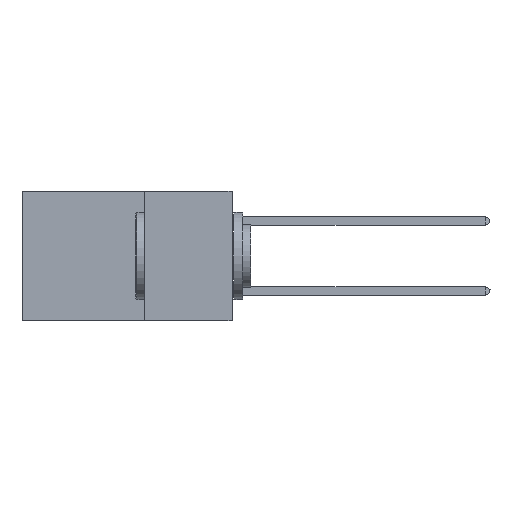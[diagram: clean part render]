
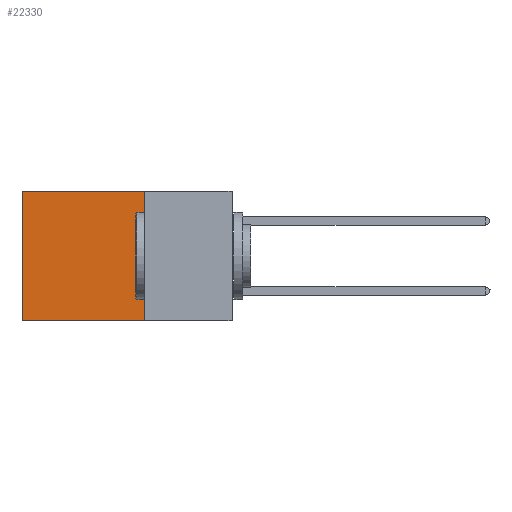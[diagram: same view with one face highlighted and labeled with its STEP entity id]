
A CAD part, left-side view. The second image highlights one B-rep face of the part: STEP entity #22330.
In plain terms, the highlighted planar face has unit normal (-1, 0, 0).
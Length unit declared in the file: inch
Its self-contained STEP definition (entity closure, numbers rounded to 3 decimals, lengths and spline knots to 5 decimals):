
#2095 = FACE_OUTER_BOUND ( 'NONE', #20787, .T. ) ;
#2292 = VECTOR ( 'NONE', #25020, 39.37008 ) ;
#3096 = VERTEX_POINT ( 'NONE', #30929 ) ;
#3463 = ORIENTED_EDGE ( 'NONE', *, *, #4629, .T. ) ;
#4629 = EDGE_CURVE ( 'NONE', #15099, #29458, #5696, .T. ) ;
#5671 = EDGE_CURVE ( 'NONE', #11451, #3096, #12783, .T. ) ;
#5696 = LINE ( 'NONE', #11235, #33436 ) ;
#7791 = CARTESIAN_POINT ( 'NONE',  ( 0.2875, 0.6, 0. ) ) ;
#9278 = VECTOR ( 'NONE', #15399, 39.37008 ) ;
#11235 = CARTESIAN_POINT ( 'NONE',  ( 0.2875, 0.25, 0. ) ) ;
#11451 = VERTEX_POINT ( 'NONE', #31086 ) ;
#12123 = CARTESIAN_POINT ( 'NONE',  ( 0.2875, 0.25, 0. ) ) ;
#12783 = LINE ( 'NONE', #19644, #2292 ) ;
#15099 = VERTEX_POINT ( 'NONE', #16363 ) ;
#15133 = DIRECTION ( 'NONE',  ( 0., 0., -1. ) ) ;
#15399 = DIRECTION ( 'NONE',  ( 0., 0., -1. ) ) ;
#16363 = CARTESIAN_POINT ( 'NONE',  ( 0.2875, 0.25, 0. ) ) ;
#17173 = DIRECTION ( 'NONE',  ( 0., 1., 0. ) ) ;
#17431 = ORIENTED_EDGE ( 'NONE', *, *, #31615, .T. ) ;
#19644 = CARTESIAN_POINT ( 'NONE',  ( 0.2875, 0.25, -0.37 ) ) ;
#20787 = EDGE_LOOP ( 'NONE', ( #17431, #24571, #23702, #3463 ) ) ;
#22330 = ADVANCED_FACE ( 'NONE', ( #2095 ), #25903, .F. ) ;
#22927 = DIRECTION ( 'NONE',  ( 1., 0., 0. ) ) ;
#23702 = ORIENTED_EDGE ( 'NONE', *, *, #30603, .F. ) ;
#24571 = ORIENTED_EDGE ( 'NONE', *, *, #5671, .F. ) ;
#25020 = DIRECTION ( 'NONE',  ( 0., 1., 0. ) ) ;
#25187 = VECTOR ( 'NONE', #26827, 39.37008 ) ;
#25903 = PLANE ( 'NONE',  #26740 ) ;
#26740 = AXIS2_PLACEMENT_3D ( 'NONE', #12123, #22927, #15133 ) ;
#26827 = DIRECTION ( 'NONE',  ( 0., 0., -1. ) ) ;
#26907 = LINE ( 'NONE', #31503, #9278 ) ;
#29458 = VERTEX_POINT ( 'NONE', #31950 ) ;
#30603 = EDGE_CURVE ( 'NONE', #15099, #11451, #26907, .T. ) ;
#30929 = CARTESIAN_POINT ( 'NONE',  ( 0.2875, 0.6, -0.37 ) ) ;
#31086 = CARTESIAN_POINT ( 'NONE',  ( 0.2875, 0.25, -0.37 ) ) ;
#31503 = CARTESIAN_POINT ( 'NONE',  ( 0.2875, 0.25, 0. ) ) ;
#31615 = EDGE_CURVE ( 'NONE', #29458, #3096, #32274, .T. ) ;
#31950 = CARTESIAN_POINT ( 'NONE',  ( 0.2875, 0.6, 0. ) ) ;
#32274 = LINE ( 'NONE', #7791, #25187 ) ;
#33436 = VECTOR ( 'NONE', #17173, 39.37008 ) ;
